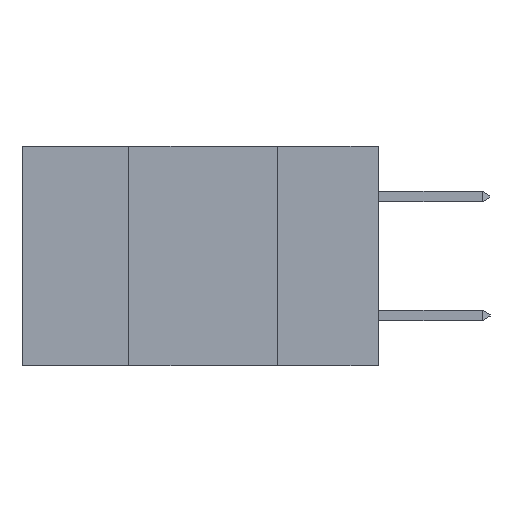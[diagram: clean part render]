
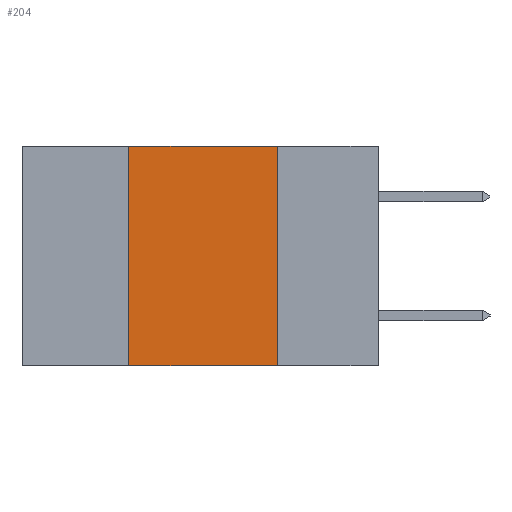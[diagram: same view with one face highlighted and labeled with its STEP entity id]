
A CAD part, left-side view. The second image highlights one B-rep face of the part: STEP entity #204.
In plain terms, the highlighted planar face has unit normal (-1, 0, 0).
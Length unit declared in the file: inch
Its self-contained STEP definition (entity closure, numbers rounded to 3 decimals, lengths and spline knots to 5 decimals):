
#204 = ADVANCED_FACE ( 'NONE', ( #18438 ), #20254, .F. ) ;
#2628 = CARTESIAN_POINT ( 'NONE',  ( 0., 0.42, -0.37 ) ) ;
#3111 = EDGE_CURVE ( 'NONE', #16661, #4958, #11822, .T. ) ;
#3201 = LINE ( 'NONE', #3678, #11302 ) ;
#3678 = CARTESIAN_POINT ( 'NONE',  ( 0., 0.17, -0.37 ) ) ;
#4835 = CARTESIAN_POINT ( 'NONE',  ( 0., 0.17, -0.37 ) ) ;
#4958 = VERTEX_POINT ( 'NONE', #18912 ) ;
#5238 = CARTESIAN_POINT ( 'NONE',  ( 0., 0.6, -0.37 ) ) ;
#5575 = EDGE_CURVE ( 'NONE', #17472, #18990, #17322, .T. ) ;
#6954 = DIRECTION ( 'NONE',  ( 0., -1., 0. ) ) ;
#7157 = DIRECTION ( 'NONE',  ( 0., 0., -1. ) ) ;
#7494 = LINE ( 'NONE', #2628, #16056 ) ;
#9317 = ORIENTED_EDGE ( 'NONE', *, *, #3111, .F. ) ;
#10121 = AXIS2_PLACEMENT_3D ( 'NONE', #11132, #17140, #16921 ) ;
#11086 = EDGE_LOOP ( 'NONE', ( #16038, #9317, #14532, #20845 ) ) ;
#11132 = CARTESIAN_POINT ( 'NONE',  ( 0., 0.6, 0. ) ) ;
#11302 = VECTOR ( 'NONE', #7157, 39.37008 ) ;
#11822 = LINE ( 'NONE', #15072, #12876 ) ;
#12278 = VECTOR ( 'NONE', #6954, 39.37008 ) ;
#12876 = VECTOR ( 'NONE', #14949, 39.37008 ) ;
#14532 = ORIENTED_EDGE ( 'NONE', *, *, #15483, .F. ) ;
#14535 = CARTESIAN_POINT ( 'NONE',  ( 0., 0.42, -0.37 ) ) ;
#14574 = CARTESIAN_POINT ( 'NONE',  ( 0., 0.42, 0. ) ) ;
#14949 = DIRECTION ( 'NONE',  ( 0., -1., 0. ) ) ;
#15072 = CARTESIAN_POINT ( 'NONE',  ( 0., 0.6, 0. ) ) ;
#15483 = EDGE_CURVE ( 'NONE', #17472, #16661, #7494, .T. ) ;
#16038 = ORIENTED_EDGE ( 'NONE', *, *, #21661, .F. ) ;
#16056 = VECTOR ( 'NONE', #18029, 39.37008 ) ;
#16661 = VERTEX_POINT ( 'NONE', #14574 ) ;
#16921 = DIRECTION ( 'NONE',  ( 0., 0., -1. ) ) ;
#17140 = DIRECTION ( 'NONE',  ( 1., 0., 0. ) ) ;
#17322 = LINE ( 'NONE', #5238, #12278 ) ;
#17472 = VERTEX_POINT ( 'NONE', #14535 ) ;
#18029 = DIRECTION ( 'NONE',  ( 0., 0., 1. ) ) ;
#18438 = FACE_OUTER_BOUND ( 'NONE', #11086, .T. ) ;
#18912 = CARTESIAN_POINT ( 'NONE',  ( 0., 0.17, 0. ) ) ;
#18990 = VERTEX_POINT ( 'NONE', #4835 ) ;
#20254 = PLANE ( 'NONE',  #10121 ) ;
#20845 = ORIENTED_EDGE ( 'NONE', *, *, #5575, .T. ) ;
#21661 = EDGE_CURVE ( 'NONE', #4958, #18990, #3201, .T. ) ;
